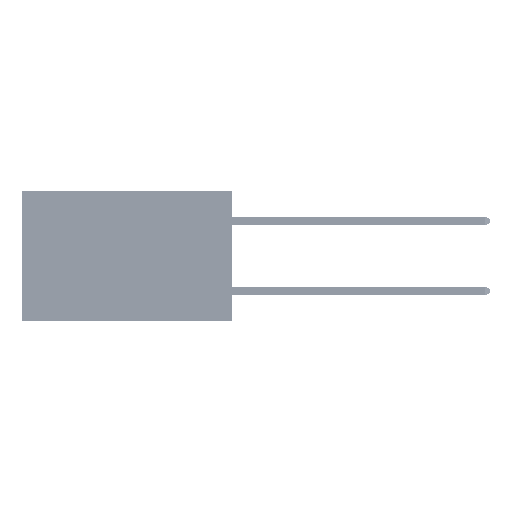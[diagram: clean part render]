
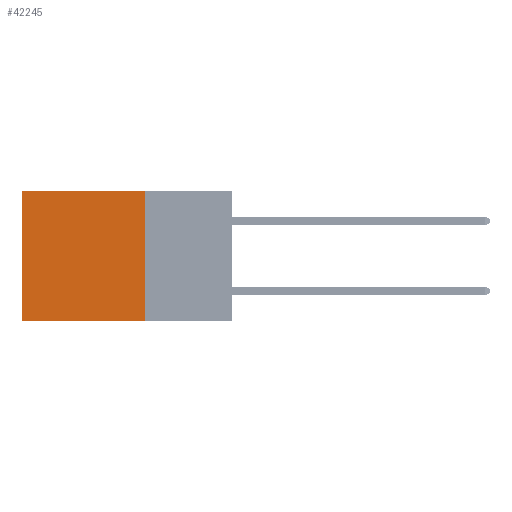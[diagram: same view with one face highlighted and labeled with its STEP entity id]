
A CAD part, left-side view. The second image highlights one B-rep face of the part: STEP entity #42245.
In plain terms, the highlighted planar face has unit normal (-1, 0, 0).
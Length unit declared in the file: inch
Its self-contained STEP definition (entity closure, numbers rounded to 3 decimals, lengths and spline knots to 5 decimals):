
#420 = ORIENTED_EDGE ( 'NONE', *, *, #33390, .F. ) ;
#541 = VECTOR ( 'NONE', #14425, 39.37008 ) ;
#547 = EDGE_CURVE ( 'NONE', #27593, #46229, #30631, .T. ) ;
#830 = DIRECTION ( 'NONE',  ( 0., 0., -1. ) ) ;
#1245 = LINE ( 'NONE', #38327, #40919 ) ;
#1417 = ORIENTED_EDGE ( 'NONE', *, *, #547, .F. ) ;
#2310 = PLANE ( 'NONE',  #25532 ) ;
#3461 = CARTESIAN_POINT ( 'NONE',  ( 0.2875, 0.25, 0. ) ) ;
#6207 = CARTESIAN_POINT ( 'NONE',  ( 0.2875, 0.25, 0. ) ) ;
#9404 = VERTEX_POINT ( 'NONE', #38727 ) ;
#9907 = DIRECTION ( 'NONE',  ( 0., 0., -1. ) ) ;
#10396 = CARTESIAN_POINT ( 'NONE',  ( 0.2875, 0.6, -0.37 ) ) ;
#12812 = VERTEX_POINT ( 'NONE', #39468 ) ;
#14425 = DIRECTION ( 'NONE',  ( 0., 1., 0. ) ) ;
#14922 = ORIENTED_EDGE ( 'NONE', *, *, #17564, .T. ) ;
#17564 = EDGE_CURVE ( 'NONE', #9404, #12812, #1245, .T. ) ;
#19176 = EDGE_CURVE ( 'NONE', #12812, #46229, #42831, .T. ) ;
#21181 = VECTOR ( 'NONE', #830, 39.37008 ) ;
#21788 = DIRECTION ( 'NONE',  ( 1., 0., 0. ) ) ;
#23420 = VECTOR ( 'NONE', #38197, 39.37008 ) ;
#25532 = AXIS2_PLACEMENT_3D ( 'NONE', #6207, #21788, #9907 ) ;
#27593 = VERTEX_POINT ( 'NONE', #29444 ) ;
#29444 = CARTESIAN_POINT ( 'NONE',  ( 0.2875, 0.25, -0.37 ) ) ;
#30631 = LINE ( 'NONE', #45322, #541 ) ;
#31319 = ORIENTED_EDGE ( 'NONE', *, *, #19176, .T. ) ;
#33390 = EDGE_CURVE ( 'NONE', #9404, #27593, #44459, .T. ) ;
#38197 = DIRECTION ( 'NONE',  ( 0., 0., -1. ) ) ;
#38327 = CARTESIAN_POINT ( 'NONE',  ( 0.2875, 0.25, 0. ) ) ;
#38727 = CARTESIAN_POINT ( 'NONE',  ( 0.2875, 0.25, 0. ) ) ;
#39288 = CARTESIAN_POINT ( 'NONE',  ( 0.2875, 0.6, 0. ) ) ;
#39468 = CARTESIAN_POINT ( 'NONE',  ( 0.2875, 0.6, 0. ) ) ;
#40919 = VECTOR ( 'NONE', #42246, 39.37008 ) ;
#42245 = ADVANCED_FACE ( 'NONE', ( #43425 ), #2310, .F. ) ;
#42246 = DIRECTION ( 'NONE',  ( 0., 1., 0. ) ) ;
#42831 = LINE ( 'NONE', #39288, #21181 ) ;
#43425 = FACE_OUTER_BOUND ( 'NONE', #49251, .T. ) ;
#44459 = LINE ( 'NONE', #3461, #23420 ) ;
#45322 = CARTESIAN_POINT ( 'NONE',  ( 0.2875, 0.25, -0.37 ) ) ;
#46229 = VERTEX_POINT ( 'NONE', #10396 ) ;
#49251 = EDGE_LOOP ( 'NONE', ( #31319, #1417, #420, #14922 ) ) ;
